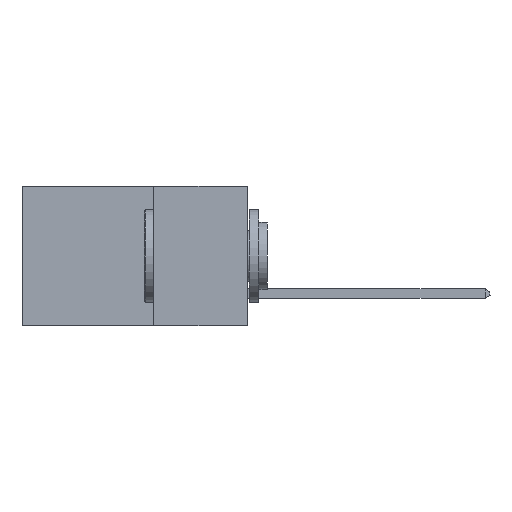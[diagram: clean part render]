
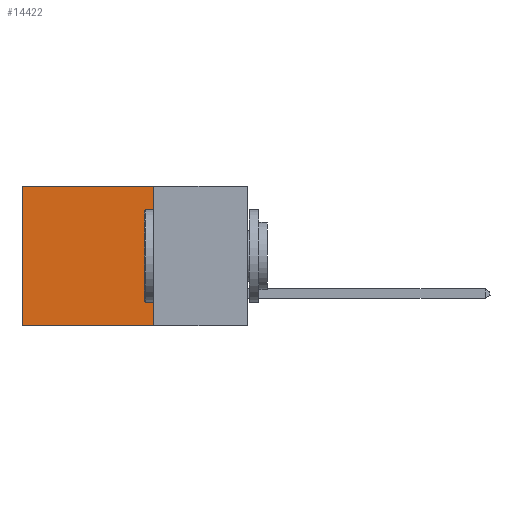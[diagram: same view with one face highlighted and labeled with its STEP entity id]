
A CAD part, left-side view. The second image highlights one B-rep face of the part: STEP entity #14422.
In plain terms, the highlighted planar face has unit normal (-1, 0, 0).
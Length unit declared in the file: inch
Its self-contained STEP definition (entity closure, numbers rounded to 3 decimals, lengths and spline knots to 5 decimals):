
#198 = CARTESIAN_POINT ( 'NONE',  ( 0.298, 0.6, -0.37 ) ) ;
#654 = VECTOR ( 'NONE', #14197, 39.37008 ) ;
#869 = ORIENTED_EDGE ( 'NONE', *, *, #5473, .F. ) ;
#1110 = AXIS2_PLACEMENT_3D ( 'NONE', #12200, #15513, #20064 ) ;
#1384 = VERTEX_POINT ( 'NONE', #198 ) ;
#2482 = FACE_OUTER_BOUND ( 'NONE', #19585, .T. ) ;
#2795 = VECTOR ( 'NONE', #16841, 39.37008 ) ;
#3787 = CARTESIAN_POINT ( 'NONE',  ( 0.298, 0.25, -0.37 ) ) ;
#3790 = LINE ( 'NONE', #10133, #2795 ) ;
#4337 = LINE ( 'NONE', #5043, #654 ) ;
#5043 = CARTESIAN_POINT ( 'NONE',  ( 0.298, 0.25, 0. ) ) ;
#5168 = VERTEX_POINT ( 'NONE', #3787 ) ;
#5473 = EDGE_CURVE ( 'NONE', #13771, #5168, #4337, .T. ) ;
#6433 = ORIENTED_EDGE ( 'NONE', *, *, #15630, .T. ) ;
#6668 = CARTESIAN_POINT ( 'NONE',  ( 0.298, 0.25, 0. ) ) ;
#9642 = EDGE_CURVE ( 'NONE', #13771, #19363, #20150, .T. ) ;
#10133 = CARTESIAN_POINT ( 'NONE',  ( 0.298, 0.6, 0. ) ) ;
#10490 = ORIENTED_EDGE ( 'NONE', *, *, #18056, .F. ) ;
#10902 = DIRECTION ( 'NONE',  ( 0., 1., 0. ) ) ;
#12200 = CARTESIAN_POINT ( 'NONE',  ( 0.298, 0.25, 0. ) ) ;
#12633 = CARTESIAN_POINT ( 'NONE',  ( 0.298, 0.6, 0. ) ) ;
#13771 = VERTEX_POINT ( 'NONE', #13968 ) ;
#13968 = CARTESIAN_POINT ( 'NONE',  ( 0.298, 0.25, 0. ) ) ;
#14197 = DIRECTION ( 'NONE',  ( 0., 0., -1. ) ) ;
#14422 = ADVANCED_FACE ( 'NONE', ( #2482 ), #15365, .F. ) ;
#15365 = PLANE ( 'NONE',  #1110 ) ;
#15513 = DIRECTION ( 'NONE',  ( 1., 0., 0. ) ) ;
#15630 = EDGE_CURVE ( 'NONE', #19363, #1384, #3790, .T. ) ;
#15822 = VECTOR ( 'NONE', #10902, 39.37008 ) ;
#16841 = DIRECTION ( 'NONE',  ( 0., 0., -1. ) ) ;
#16966 = CARTESIAN_POINT ( 'NONE',  ( 0.298, 0.25, -0.37 ) ) ;
#17963 = VECTOR ( 'NONE', #18941, 39.37008 ) ;
#18056 = EDGE_CURVE ( 'NONE', #5168, #1384, #19988, .T. ) ;
#18720 = ORIENTED_EDGE ( 'NONE', *, *, #9642, .T. ) ;
#18941 = DIRECTION ( 'NONE',  ( 0., 1., 0. ) ) ;
#19363 = VERTEX_POINT ( 'NONE', #12633 ) ;
#19585 = EDGE_LOOP ( 'NONE', ( #6433, #10490, #869, #18720 ) ) ;
#19988 = LINE ( 'NONE', #16966, #15822 ) ;
#20064 = DIRECTION ( 'NONE',  ( 0., 0., -1. ) ) ;
#20150 = LINE ( 'NONE', #6668, #17963 ) ;
